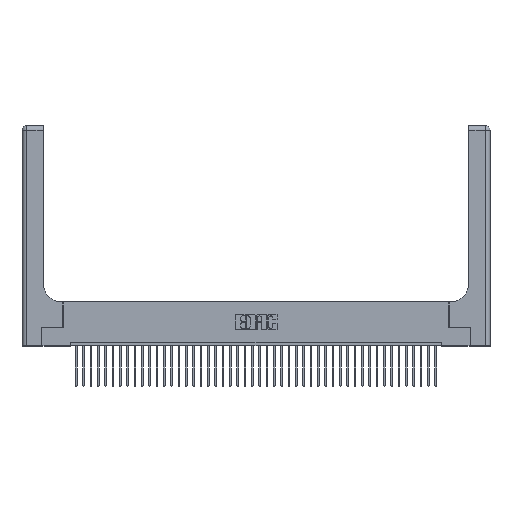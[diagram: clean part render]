
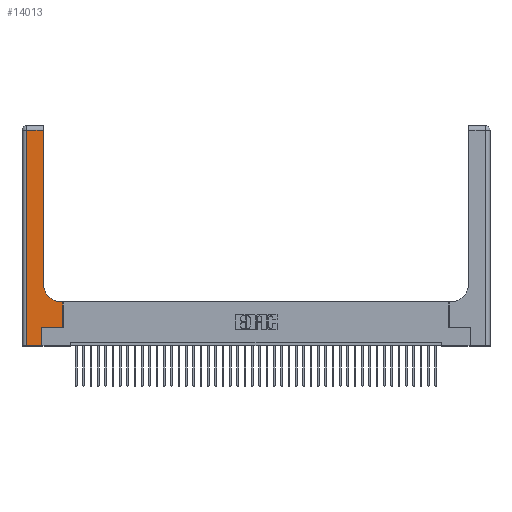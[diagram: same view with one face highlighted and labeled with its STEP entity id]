
A CAD part, top view. The second image highlights one B-rep face of the part: STEP entity #14013.
In plain terms, the highlighted planar face has unit normal (0, 0, 1).
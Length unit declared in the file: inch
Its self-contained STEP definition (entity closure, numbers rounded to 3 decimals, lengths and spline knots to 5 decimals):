
#1579 = CARTESIAN_POINT ( 'NONE',  ( 0.269, 0., 0.37 ) ) ;
#1713 = ORIENTED_EDGE ( 'NONE', *, *, #37971, .T. ) ;
#2145 = EDGE_CURVE ( 'NONE', #20434, #23981, #29748, .T. ) ;
#2212 = EDGE_CURVE ( 'NONE', #32294, #6960, #21320, .T. ) ;
#2465 = DIRECTION ( 'NONE',  ( 1., 0., 0. ) ) ;
#3377 = CARTESIAN_POINT ( 'NONE',  ( 0.5585, 0.25, 0.37 ) ) ;
#3560 = EDGE_CURVE ( 'NONE', #4503, #35674, #37829, .T. ) ;
#4349 = EDGE_CURVE ( 'NONE', #35674, #19491, #25664, .T. ) ;
#4503 = VERTEX_POINT ( 'NONE', #30843 ) ;
#5147 = DIRECTION ( 'NONE',  ( -1., 0., 0. ) ) ;
#6357 = LINE ( 'NONE', #12971, #17407 ) ;
#6960 = VERTEX_POINT ( 'NONE', #3377 ) ;
#8177 = DIRECTION ( 'NONE',  ( 0., 0., -1. ) ) ;
#8400 = CARTESIAN_POINT ( 'NONE',  ( 0.06, 3., 0.37 ) ) ;
#8406 = DIRECTION ( 'NONE',  ( 0., 1., 0. ) ) ;
#9806 = EDGE_CURVE ( 'NONE', #27120, #4503, #10914, .T. ) ;
#10914 = LINE ( 'NONE', #34176, #36622 ) ;
#11400 = DIRECTION ( 'NONE',  ( -1., 0., 0. ) ) ;
#11983 = AXIS2_PLACEMENT_3D ( 'NONE', #34910, #15352, #2465 ) ;
#12066 = EDGE_CURVE ( 'NONE', #26672, #32294, #40896, .T. ) ;
#12494 = ORIENTED_EDGE ( 'NONE', *, *, #2145, .T. ) ;
#12971 = CARTESIAN_POINT ( 'NONE',  ( 0.5585, 0.25, 0.37 ) ) ;
#13472 = FACE_OUTER_BOUND ( 'NONE', #15128, .T. ) ;
#13638 = VECTOR ( 'NONE', #34301, 39.37008 ) ;
#13750 = CARTESIAN_POINT ( 'NONE',  ( 0.06, 2.94, 0.37 ) ) ;
#13884 = ORIENTED_EDGE ( 'NONE', *, *, #12066, .T. ) ;
#14013 = ADVANCED_FACE ( 'NONE', ( #13472 ), #27475, .F. ) ;
#14278 = LINE ( 'NONE', #23697, #31924 ) ;
#15128 = EDGE_LOOP ( 'NONE', ( #19415, #27905, #12494, #19510, #13884, #32612, #1713, #20240, #15445 ) ) ;
#15352 = DIRECTION ( 'NONE',  ( 0., 0., -1. ) ) ;
#15445 = ORIENTED_EDGE ( 'NONE', *, *, #3560, .T. ) ;
#17034 = VECTOR ( 'NONE', #37053, 39.37008 ) ;
#17407 = VECTOR ( 'NONE', #19585, 39.37008 ) ;
#19415 = ORIENTED_EDGE ( 'NONE', *, *, #4349, .T. ) ;
#19491 = VERTEX_POINT ( 'NONE', #41296 ) ;
#19510 = ORIENTED_EDGE ( 'NONE', *, *, #40381, .T. ) ;
#19585 = DIRECTION ( 'NONE',  ( 0., 1., 0. ) ) ;
#20240 = ORIENTED_EDGE ( 'NONE', *, *, #9806, .T. ) ;
#20434 = VERTEX_POINT ( 'NONE', #13750 ) ;
#20952 = DIRECTION ( 'NONE',  ( 1., 0., 0. ) ) ;
#21320 = LINE ( 'NONE', #33713, #22333 ) ;
#22333 = VECTOR ( 'NONE', #20952, 39.37008 ) ;
#23697 = CARTESIAN_POINT ( 'NONE',  ( 0., 2.94, 0.37 ) ) ;
#23981 = VERTEX_POINT ( 'NONE', #30089 ) ;
#24917 = AXIS2_PLACEMENT_3D ( 'NONE', #37174, #8177, #11400 ) ;
#25664 = LINE ( 'NONE', #37212, #17034 ) ;
#26009 = DIRECTION ( 'NONE',  ( 1., 0., 0. ) ) ;
#26672 = VERTEX_POINT ( 'NONE', #1579 ) ;
#26792 = LINE ( 'NONE', #32204, #41444 ) ;
#27120 = VERTEX_POINT ( 'NONE', #40247 ) ;
#27475 = PLANE ( 'NONE',  #24917 ) ;
#27905 = ORIENTED_EDGE ( 'NONE', *, *, #28176, .T. ) ;
#28176 = EDGE_CURVE ( 'NONE', #19491, #20434, #14278, .T. ) ;
#29748 = LINE ( 'NONE', #8400, #13638 ) ;
#30089 = CARTESIAN_POINT ( 'NONE',  ( 0.06, 0., 0.37 ) ) ;
#30843 = CARTESIAN_POINT ( 'NONE',  ( 0.5415, 0.6, 0.37 ) ) ;
#31924 = VECTOR ( 'NONE', #40304, 39.37008 ) ;
#32204 = CARTESIAN_POINT ( 'NONE',  ( 0., 0., 0.37 ) ) ;
#32294 = VERTEX_POINT ( 'NONE', #39289 ) ;
#32612 = ORIENTED_EDGE ( 'NONE', *, *, #2212, .T. ) ;
#33713 = CARTESIAN_POINT ( 'NONE',  ( 0.269, 0.25, 0.37 ) ) ;
#33795 = VECTOR ( 'NONE', #8406, 39.37008 ) ;
#33855 = CARTESIAN_POINT ( 'NONE',  ( 0.269, 0., 0.37 ) ) ;
#34176 = CARTESIAN_POINT ( 'NONE',  ( 0.2915, 0.6, 0.37 ) ) ;
#34301 = DIRECTION ( 'NONE',  ( 0., -1., 0. ) ) ;
#34910 = CARTESIAN_POINT ( 'NONE',  ( 0.5415, 0.85, 0.37 ) ) ;
#35147 = CARTESIAN_POINT ( 'NONE',  ( 0.2915, 0.85, 0.37 ) ) ;
#35674 = VERTEX_POINT ( 'NONE', #35147 ) ;
#36622 = VECTOR ( 'NONE', #5147, 39.37008 ) ;
#37053 = DIRECTION ( 'NONE',  ( 0., 1., 0. ) ) ;
#37174 = CARTESIAN_POINT ( 'NONE',  ( 0., 3., 0.37 ) ) ;
#37212 = CARTESIAN_POINT ( 'NONE',  ( 0.2915, 3., 0.37 ) ) ;
#37829 = CIRCLE ( 'NONE', #11983, 0.25 ) ;
#37971 = EDGE_CURVE ( 'NONE', #6960, #27120, #6357, .T. ) ;
#39289 = CARTESIAN_POINT ( 'NONE',  ( 0.269, 0.25, 0.37 ) ) ;
#40247 = CARTESIAN_POINT ( 'NONE',  ( 0.5585, 0.6, 0.37 ) ) ;
#40304 = DIRECTION ( 'NONE',  ( -1., 0., 0. ) ) ;
#40381 = EDGE_CURVE ( 'NONE', #23981, #26672, #26792, .T. ) ;
#40896 = LINE ( 'NONE', #33855, #33795 ) ;
#41296 = CARTESIAN_POINT ( 'NONE',  ( 0.2915, 2.94, 0.37 ) ) ;
#41444 = VECTOR ( 'NONE', #26009, 39.37008 ) ;
